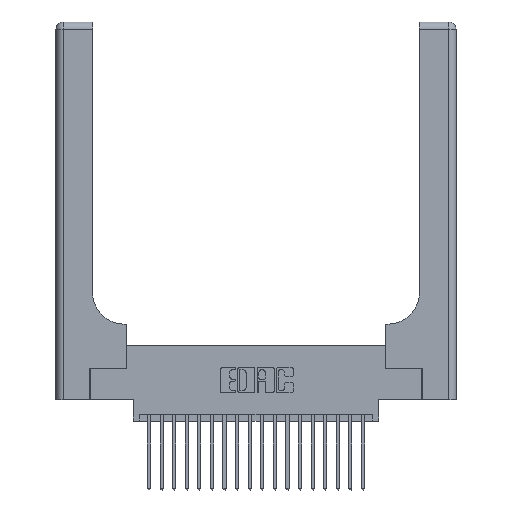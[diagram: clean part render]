
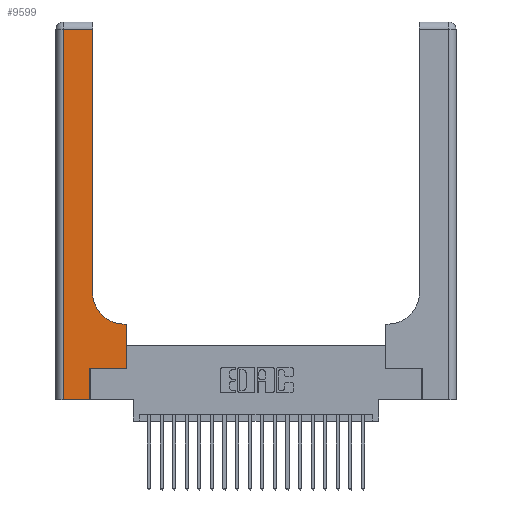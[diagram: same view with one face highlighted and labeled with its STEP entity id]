
A CAD part, top view. The second image highlights one B-rep face of the part: STEP entity #9599.
In plain terms, the highlighted planar face has unit normal (0, 0, 1).
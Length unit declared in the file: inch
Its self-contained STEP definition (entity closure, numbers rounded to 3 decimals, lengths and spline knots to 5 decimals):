
#364 = DIRECTION ( 'NONE',  ( 0., 0., -1. ) ) ;
#1276 = LINE ( 'NONE', #17676, #5976 ) ;
#1298 = ORIENTED_EDGE ( 'NONE', *, *, #7799, .T. ) ;
#1571 = DIRECTION ( 'NONE',  ( -1., 0., 0. ) ) ;
#1811 = ORIENTED_EDGE ( 'NONE', *, *, #6149, .T. ) ;
#1837 = ORIENTED_EDGE ( 'NONE', *, *, #12780, .T. ) ;
#2019 = LINE ( 'NONE', #9397, #6180 ) ;
#2194 = LINE ( 'NONE', #5937, #20371 ) ;
#2583 = CARTESIAN_POINT ( 'NONE',  ( 0.5415, 0.6, 0.37 ) ) ;
#3591 = LINE ( 'NONE', #8808, #17720 ) ;
#4199 = CARTESIAN_POINT ( 'NONE',  ( 0.5585, 0.25, 0.37 ) ) ;
#4428 = CARTESIAN_POINT ( 'NONE',  ( 0.06, 0., 0.37 ) ) ;
#5142 = CARTESIAN_POINT ( 'NONE',  ( 0.06, 3., 0.37 ) ) ;
#5354 = ORIENTED_EDGE ( 'NONE', *, *, #15931, .T. ) ;
#5937 = CARTESIAN_POINT ( 'NONE',  ( 0.269, 0., 0.37 ) ) ;
#5976 = VECTOR ( 'NONE', #15889, 39.37008 ) ;
#6149 = EDGE_CURVE ( 'NONE', #19672, #15756, #16408, .T. ) ;
#6180 = VECTOR ( 'NONE', #14742, 39.37008 ) ;
#6884 = VECTOR ( 'NONE', #6921, 39.37008 ) ;
#6921 = DIRECTION ( 'NONE',  ( 0., -1., 0. ) ) ;
#7025 = CARTESIAN_POINT ( 'NONE',  ( 0., 2.94, 0.37 ) ) ;
#7673 = CARTESIAN_POINT ( 'NONE',  ( 0.269, 0., 0.37 ) ) ;
#7795 = ORIENTED_EDGE ( 'NONE', *, *, #14043, .T. ) ;
#7799 = EDGE_CURVE ( 'NONE', #20986, #18217, #21172, .T. ) ;
#7887 = VERTEX_POINT ( 'NONE', #7673 ) ;
#8058 = CARTESIAN_POINT ( 'NONE',  ( 0., 3., 0.37 ) ) ;
#8219 = CARTESIAN_POINT ( 'NONE',  ( 0.5585, 0.6, 0.37 ) ) ;
#8462 = VECTOR ( 'NONE', #21038, 39.37008 ) ;
#8808 = CARTESIAN_POINT ( 'NONE',  ( 0.2915, 3., 0.37 ) ) ;
#9021 = CARTESIAN_POINT ( 'NONE',  ( 0.06, 2.94, 0.37 ) ) ;
#9397 = CARTESIAN_POINT ( 'NONE',  ( 0.269, 0.25, 0.37 ) ) ;
#9599 = ADVANCED_FACE ( 'NONE', ( #21392 ), #18555, .F. ) ;
#9808 = DIRECTION ( 'NONE',  ( -1., 0., 0. ) ) ;
#9898 = DIRECTION ( 'NONE',  ( 0., 1., 0. ) ) ;
#10229 = VERTEX_POINT ( 'NONE', #4428 ) ;
#10548 = EDGE_CURVE ( 'NONE', #19175, #18438, #22395, .T. ) ;
#10662 = ORIENTED_EDGE ( 'NONE', *, *, #10548, .T. ) ;
#10878 = CARTESIAN_POINT ( 'NONE',  ( 0.5415, 0.85, 0.37 ) ) ;
#11047 = LINE ( 'NONE', #22559, #15223 ) ;
#11175 = EDGE_CURVE ( 'NONE', #10229, #7887, #1276, .T. ) ;
#11225 = DIRECTION ( 'NONE',  ( 0., 1., 0. ) ) ;
#11510 = LINE ( 'NONE', #5142, #6884 ) ;
#11671 = CARTESIAN_POINT ( 'NONE',  ( 0.269, 0.25, 0.37 ) ) ;
#12666 = DIRECTION ( 'NONE',  ( 1., 0., 0. ) ) ;
#12780 = EDGE_CURVE ( 'NONE', #15077, #19672, #2019, .T. ) ;
#13373 = CARTESIAN_POINT ( 'NONE',  ( 0.5585, 0.25, 0.37 ) ) ;
#14043 = EDGE_CURVE ( 'NONE', #15756, #20986, #11047, .T. ) ;
#14634 = EDGE_CURVE ( 'NONE', #18217, #19175, #3591, .T. ) ;
#14742 = DIRECTION ( 'NONE',  ( 1., 0., 0. ) ) ;
#14906 = EDGE_CURVE ( 'NONE', #7887, #15077, #2194, .T. ) ;
#15077 = VERTEX_POINT ( 'NONE', #11671 ) ;
#15223 = VECTOR ( 'NONE', #1571, 39.37008 ) ;
#15750 = AXIS2_PLACEMENT_3D ( 'NONE', #10878, #364, #12666 ) ;
#15756 = VERTEX_POINT ( 'NONE', #8219 ) ;
#15889 = DIRECTION ( 'NONE',  ( 1., 0., 0. ) ) ;
#15914 = AXIS2_PLACEMENT_3D ( 'NONE', #8058, #20333, #9808 ) ;
#15931 = EDGE_CURVE ( 'NONE', #18438, #10229, #11510, .T. ) ;
#16408 = LINE ( 'NONE', #13373, #19912 ) ;
#16673 = EDGE_LOOP ( 'NONE', ( #19643, #10662, #5354, #22136, #21693, #1837, #1811, #7795, #1298 ) ) ;
#17324 = CARTESIAN_POINT ( 'NONE',  ( 0.2915, 0.85, 0.37 ) ) ;
#17676 = CARTESIAN_POINT ( 'NONE',  ( 0., 0., 0.37 ) ) ;
#17720 = VECTOR ( 'NONE', #21047, 39.37008 ) ;
#18217 = VERTEX_POINT ( 'NONE', #17324 ) ;
#18438 = VERTEX_POINT ( 'NONE', #9021 ) ;
#18555 = PLANE ( 'NONE',  #15914 ) ;
#18716 = CARTESIAN_POINT ( 'NONE',  ( 0.2915, 2.94, 0.37 ) ) ;
#19175 = VERTEX_POINT ( 'NONE', #18716 ) ;
#19643 = ORIENTED_EDGE ( 'NONE', *, *, #14634, .T. ) ;
#19672 = VERTEX_POINT ( 'NONE', #4199 ) ;
#19912 = VECTOR ( 'NONE', #9898, 39.37008 ) ;
#20333 = DIRECTION ( 'NONE',  ( 0., 0., -1. ) ) ;
#20371 = VECTOR ( 'NONE', #11225, 39.37008 ) ;
#20986 = VERTEX_POINT ( 'NONE', #2583 ) ;
#21038 = DIRECTION ( 'NONE',  ( -1., 0., 0. ) ) ;
#21047 = DIRECTION ( 'NONE',  ( 0., 1., 0. ) ) ;
#21172 = CIRCLE ( 'NONE', #15750, 0.25 ) ;
#21392 = FACE_OUTER_BOUND ( 'NONE', #16673, .T. ) ;
#21693 = ORIENTED_EDGE ( 'NONE', *, *, #14906, .T. ) ;
#22136 = ORIENTED_EDGE ( 'NONE', *, *, #11175, .T. ) ;
#22395 = LINE ( 'NONE', #7025, #8462 ) ;
#22559 = CARTESIAN_POINT ( 'NONE',  ( 0.2915, 0.6, 0.37 ) ) ;
